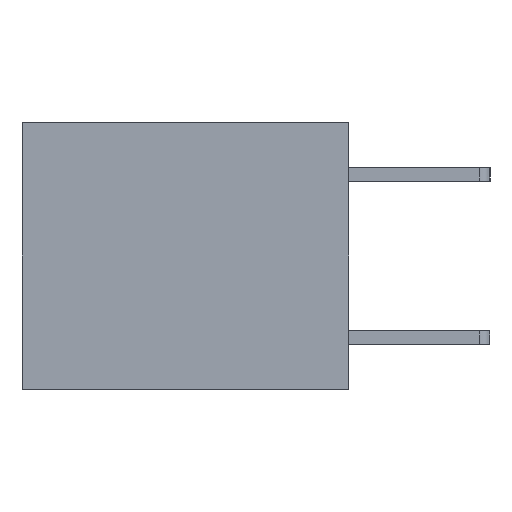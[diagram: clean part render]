
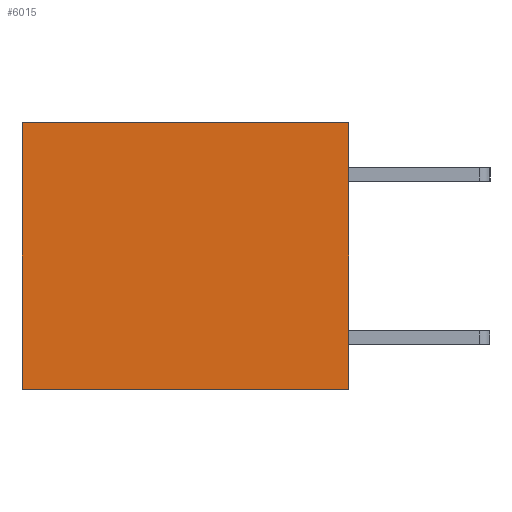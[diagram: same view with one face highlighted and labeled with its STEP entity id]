
A CAD part, left-side view. The second image highlights one B-rep face of the part: STEP entity #6015.
In plain terms, the highlighted planar face has unit normal (-1, 0, 0).
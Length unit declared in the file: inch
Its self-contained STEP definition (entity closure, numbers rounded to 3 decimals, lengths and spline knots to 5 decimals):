
#86 = CARTESIAN_POINT ( 'NONE',  ( 0.3165, 0.6, -0.49 ) ) ;
#269 = VERTEX_POINT ( 'NONE', #771 ) ;
#528 = LINE ( 'NONE', #6714, #4370 ) ;
#597 = EDGE_CURVE ( 'NONE', #269, #5623, #528, .T. ) ;
#628 = VERTEX_POINT ( 'NONE', #6038 ) ;
#771 = CARTESIAN_POINT ( 'NONE',  ( 0.3165, 0., 0. ) ) ;
#1339 = CARTESIAN_POINT ( 'NONE',  ( 0.3165, 0., -0.49 ) ) ;
#2175 = EDGE_CURVE ( 'NONE', #269, #10626, #12235, .T. ) ;
#2456 = PLANE ( 'NONE',  #9178 ) ;
#2813 = VECTOR ( 'NONE', #10129, 39.37008 ) ;
#3275 = ORIENTED_EDGE ( 'NONE', *, *, #12198, .T. ) ;
#3694 = CARTESIAN_POINT ( 'NONE',  ( 0.3165, 0., -0.49 ) ) ;
#3700 = ORIENTED_EDGE ( 'NONE', *, *, #2175, .T. ) ;
#4160 = CARTESIAN_POINT ( 'NONE',  ( 0.3165, 0., -0.49 ) ) ;
#4370 = VECTOR ( 'NONE', #13472, 39.37008 ) ;
#4470 = DIRECTION ( 'NONE',  ( 1., 0., 0. ) ) ;
#4490 = CARTESIAN_POINT ( 'NONE',  ( 0.3165, 0.6, 0. ) ) ;
#5145 = LINE ( 'NONE', #86, #11036 ) ;
#5623 = VERTEX_POINT ( 'NONE', #4160 ) ;
#6015 = ADVANCED_FACE ( 'NONE', ( #13564 ), #2456, .F. ) ;
#6038 = CARTESIAN_POINT ( 'NONE',  ( 0.3165, 0.6, -0.49 ) ) ;
#6585 = CARTESIAN_POINT ( 'NONE',  ( 0.3165, 0., 0. ) ) ;
#6714 = CARTESIAN_POINT ( 'NONE',  ( 0.3165, 0., -0.49 ) ) ;
#7717 = VECTOR ( 'NONE', #9726, 39.37008 ) ;
#7825 = ORIENTED_EDGE ( 'NONE', *, *, #10239, .F. ) ;
#9178 = AXIS2_PLACEMENT_3D ( 'NONE', #1339, #4470, #12130 ) ;
#9726 = DIRECTION ( 'NONE',  ( 0., 1., 0. ) ) ;
#10129 = DIRECTION ( 'NONE',  ( 0., 1., 0. ) ) ;
#10239 = EDGE_CURVE ( 'NONE', #5623, #628, #10455, .T. ) ;
#10455 = LINE ( 'NONE', #3694, #7717 ) ;
#10626 = VERTEX_POINT ( 'NONE', #4490 ) ;
#10679 = DIRECTION ( 'NONE',  ( 0., 0., -1. ) ) ;
#11036 = VECTOR ( 'NONE', #10679, 39.37008 ) ;
#12130 = DIRECTION ( 'NONE',  ( 0., 0., -1. ) ) ;
#12198 = EDGE_CURVE ( 'NONE', #10626, #628, #5145, .T. ) ;
#12235 = LINE ( 'NONE', #6585, #2813 ) ;
#13472 = DIRECTION ( 'NONE',  ( 0., 0., -1. ) ) ;
#13564 = FACE_OUTER_BOUND ( 'NONE', #13773, .T. ) ;
#13571 = ORIENTED_EDGE ( 'NONE', *, *, #597, .F. ) ;
#13773 = EDGE_LOOP ( 'NONE', ( #3275, #7825, #13571, #3700 ) ) ;
